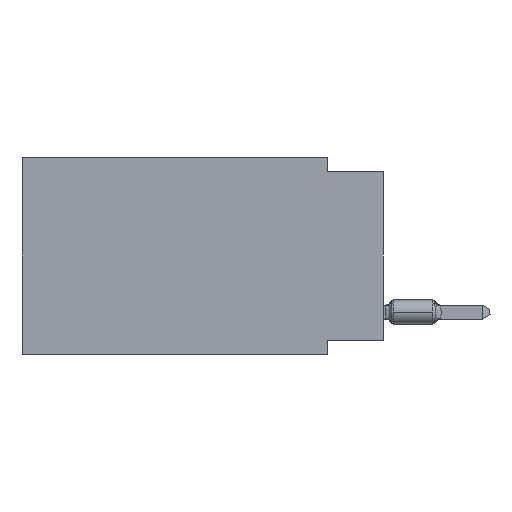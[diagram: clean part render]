
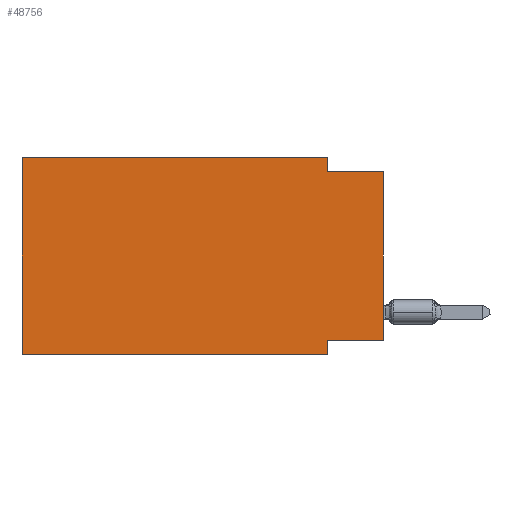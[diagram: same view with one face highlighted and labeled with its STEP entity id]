
A CAD part, left-side view. The second image highlights one B-rep face of the part: STEP entity #48756.
In plain terms, the highlighted planar face has unit normal (-1, 0, 0).
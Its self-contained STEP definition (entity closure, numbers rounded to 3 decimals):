
#221 = VECTOR ( 'NONE', #25086, 1000. ) ;
#816 = DIRECTION ( 'NONE',  ( 0., 0., -1. ) ) ;
#2604 = LINE ( 'NONE', #9385, #26129 ) ;
#2614 = VERTEX_POINT ( 'NONE', #47286 ) ;
#3071 = CARTESIAN_POINT ( 'NONE',  ( 0., 16.383, -8.89 ) ) ;
#3851 = CARTESIAN_POINT ( 'NONE',  ( 0., 2.54, 0. ) ) ;
#4831 = LINE ( 'NONE', #3851, #19086 ) ;
#5694 = VECTOR ( 'NONE', #12350, 1000. ) ;
#7391 = CARTESIAN_POINT ( 'NONE',  ( 0., 16.383, 0. ) ) ;
#8122 = CARTESIAN_POINT ( 'NONE',  ( 0., 2.54, -8.255 ) ) ;
#9385 = CARTESIAN_POINT ( 'NONE',  ( 0., 16.383, 0. ) ) ;
#9633 = CARTESIAN_POINT ( 'NONE',  ( 0., 2.54, -8.89 ) ) ;
#9767 = LINE ( 'NONE', #43670, #221 ) ;
#9782 = CARTESIAN_POINT ( 'NONE',  ( 0., 2.54, -8.89 ) ) ;
#11583 = LINE ( 'NONE', #15348, #42856 ) ;
#12350 = DIRECTION ( 'NONE',  ( 0., 1., 0. ) ) ;
#13994 = CARTESIAN_POINT ( 'NONE',  ( 0., 16.383, -8.89 ) ) ;
#15207 = CARTESIAN_POINT ( 'NONE',  ( 0., 2.54, 0. ) ) ;
#15244 = LINE ( 'NONE', #35549, #36145 ) ;
#15348 = CARTESIAN_POINT ( 'NONE',  ( 0., 0., 0. ) ) ;
#15674 = DIRECTION ( 'NONE',  ( 0., 0., -1. ) ) ;
#16612 = ORIENTED_EDGE ( 'NONE', *, *, #35894, .F. ) ;
#17269 = EDGE_CURVE ( 'NONE', #28657, #2614, #11583, .T. ) ;
#17435 = DIRECTION ( 'NONE',  ( 0., -1., 0. ) ) ;
#19086 = VECTOR ( 'NONE', #816, 1000. ) ;
#19551 = EDGE_LOOP ( 'NONE', ( #27724, #25542, #38162, #44966, #16612, #22012, #39679, #49574 ) ) ;
#22012 = ORIENTED_EDGE ( 'NONE', *, *, #36554, .T. ) ;
#22258 = EDGE_CURVE ( 'NONE', #24761, #33402, #4831, .T. ) ;
#24761 = VERTEX_POINT ( 'NONE', #15207 ) ;
#24856 = VECTOR ( 'NONE', #36398, 1000. ) ;
#25086 = DIRECTION ( 'NONE',  ( 0., 0., 1. ) ) ;
#25542 = ORIENTED_EDGE ( 'NONE', *, *, #33552, .F. ) ;
#26129 = VECTOR ( 'NONE', #17435, 1000. ) ;
#26381 = VERTEX_POINT ( 'NONE', #30455 ) ;
#27724 = ORIENTED_EDGE ( 'NONE', *, *, #17269, .T. ) ;
#28510 = DIRECTION ( 'NONE',  ( 0., -1., 0. ) ) ;
#28657 = VERTEX_POINT ( 'NONE', #29137 ) ;
#29137 = CARTESIAN_POINT ( 'NONE',  ( 0., 0., -8.255 ) ) ;
#29294 = DIRECTION ( 'NONE',  ( 0., -1., 0. ) ) ;
#30455 = CARTESIAN_POINT ( 'NONE',  ( 0., 16.383, 0. ) ) ;
#30985 = PLANE ( 'NONE',  #48710 ) ;
#31418 = LINE ( 'NONE', #31919, #5694 ) ;
#31919 = CARTESIAN_POINT ( 'NONE',  ( 0., 0., -8.255 ) ) ;
#33402 = VERTEX_POINT ( 'NONE', #36670 ) ;
#33552 = EDGE_CURVE ( 'NONE', #33402, #2614, #15244, .T. ) ;
#35549 = CARTESIAN_POINT ( 'NONE',  ( 0., 0., -0.635 ) ) ;
#35650 = VERTEX_POINT ( 'NONE', #9633 ) ;
#35894 = EDGE_CURVE ( 'NONE', #40290, #26381, #9767, .T. ) ;
#36145 = VECTOR ( 'NONE', #28510, 1000. ) ;
#36398 = DIRECTION ( 'NONE',  ( 0., 0., -1. ) ) ;
#36554 = EDGE_CURVE ( 'NONE', #40290, #35650, #37074, .T. ) ;
#36670 = CARTESIAN_POINT ( 'NONE',  ( 0., 2.54, -0.635 ) ) ;
#37074 = LINE ( 'NONE', #13994, #38752 ) ;
#37771 = EDGE_CURVE ( 'NONE', #47758, #35650, #45363, .T. ) ;
#38162 = ORIENTED_EDGE ( 'NONE', *, *, #22258, .F. ) ;
#38752 = VECTOR ( 'NONE', #29294, 1000. ) ;
#39679 = ORIENTED_EDGE ( 'NONE', *, *, #37771, .F. ) ;
#40290 = VERTEX_POINT ( 'NONE', #3071 ) ;
#40480 = EDGE_CURVE ( 'NONE', #28657, #47758, #31418, .T. ) ;
#42856 = VECTOR ( 'NONE', #45983, 1000. ) ;
#43670 = CARTESIAN_POINT ( 'NONE',  ( 0., 16.383, 0. ) ) ;
#44932 = EDGE_CURVE ( 'NONE', #26381, #24761, #2604, .T. ) ;
#44966 = ORIENTED_EDGE ( 'NONE', *, *, #44932, .F. ) ;
#45322 = FACE_OUTER_BOUND ( 'NONE', #19551, .T. ) ;
#45363 = LINE ( 'NONE', #9782, #24856 ) ;
#45983 = DIRECTION ( 'NONE',  ( 0., 0., 1. ) ) ;
#46306 = DIRECTION ( 'NONE',  ( 1., 0., 0. ) ) ;
#47286 = CARTESIAN_POINT ( 'NONE',  ( 0., 0., -0.635 ) ) ;
#47758 = VERTEX_POINT ( 'NONE', #8122 ) ;
#48710 = AXIS2_PLACEMENT_3D ( 'NONE', #7391, #46306, #15674 ) ;
#48756 = ADVANCED_FACE ( 'NONE', ( #45322 ), #30985, .F. ) ;
#49574 = ORIENTED_EDGE ( 'NONE', *, *, #40480, .F. ) ;
